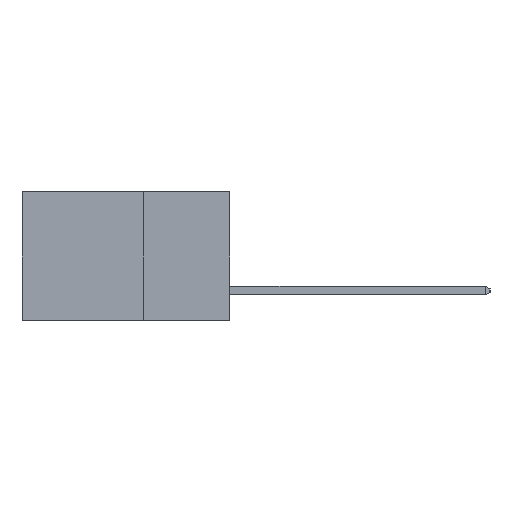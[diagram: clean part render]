
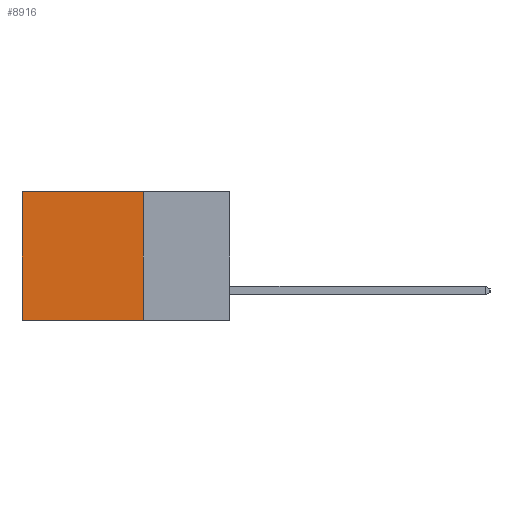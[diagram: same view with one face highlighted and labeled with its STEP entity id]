
A CAD part, left-side view. The second image highlights one B-rep face of the part: STEP entity #8916.
In plain terms, the highlighted planar face has unit normal (-1, 0, 0).
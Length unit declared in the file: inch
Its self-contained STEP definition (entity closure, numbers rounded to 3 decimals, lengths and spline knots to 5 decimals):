
#143 = DIRECTION ( 'NONE',  ( 0., 0., -1. ) ) ;
#251 = VERTEX_POINT ( 'NONE', #4258 ) ;
#1482 = EDGE_LOOP ( 'NONE', ( #3421, #2006, #2745, #1930 ) ) ;
#1563 = AXIS2_PLACEMENT_3D ( 'NONE', #13508, #4951, #7120 ) ;
#1855 = DIRECTION ( 'NONE',  ( 0., 1., 0. ) ) ;
#1930 = ORIENTED_EDGE ( 'NONE', *, *, #9659, .T. ) ;
#2006 = ORIENTED_EDGE ( 'NONE', *, *, #9370, .F. ) ;
#2319 = VECTOR ( 'NONE', #2576, 39.37008 ) ;
#2576 = DIRECTION ( 'NONE',  ( 0., 1., 0. ) ) ;
#2616 = VERTEX_POINT ( 'NONE', #10961 ) ;
#2745 = ORIENTED_EDGE ( 'NONE', *, *, #10788, .F. ) ;
#3421 = ORIENTED_EDGE ( 'NONE', *, *, #4397, .T. ) ;
#4176 = VECTOR ( 'NONE', #11426, 39.37008 ) ;
#4258 = CARTESIAN_POINT ( 'NONE',  ( 0.2615, 0.25, -0.37 ) ) ;
#4397 = EDGE_CURVE ( 'NONE', #7286, #8876, #6907, .T. ) ;
#4951 = DIRECTION ( 'NONE',  ( 1., 0., 0. ) ) ;
#4998 = LINE ( 'NONE', #6139, #13298 ) ;
#5422 = CARTESIAN_POINT ( 'NONE',  ( 0.2615, 0.6, -0.37 ) ) ;
#6139 = CARTESIAN_POINT ( 'NONE',  ( 0.2615, 0.25, 0. ) ) ;
#6532 = CARTESIAN_POINT ( 'NONE',  ( 0.2615, 0.25, -0.37 ) ) ;
#6907 = LINE ( 'NONE', #5422, #4176 ) ;
#7120 = DIRECTION ( 'NONE',  ( 0., 0., -1. ) ) ;
#7286 = VERTEX_POINT ( 'NONE', #9387 ) ;
#7936 = FACE_OUTER_BOUND ( 'NONE', #1482, .T. ) ;
#8876 = VERTEX_POINT ( 'NONE', #12491 ) ;
#8916 = ADVANCED_FACE ( 'NONE', ( #7936 ), #10298, .F. ) ;
#9370 = EDGE_CURVE ( 'NONE', #251, #8876, #10097, .T. ) ;
#9387 = CARTESIAN_POINT ( 'NONE',  ( 0.2615, 0.6, 0. ) ) ;
#9659 = EDGE_CURVE ( 'NONE', #2616, #7286, #4998, .T. ) ;
#10097 = LINE ( 'NONE', #11156, #2319 ) ;
#10298 = PLANE ( 'NONE',  #1563 ) ;
#10741 = VECTOR ( 'NONE', #143, 39.37008 ) ;
#10788 = EDGE_CURVE ( 'NONE', #2616, #251, #11918, .T. ) ;
#10961 = CARTESIAN_POINT ( 'NONE',  ( 0.2615, 0.25, 0. ) ) ;
#11156 = CARTESIAN_POINT ( 'NONE',  ( 0.2615, 0.25, -0.37 ) ) ;
#11426 = DIRECTION ( 'NONE',  ( 0., 0., -1. ) ) ;
#11918 = LINE ( 'NONE', #6532, #10741 ) ;
#12491 = CARTESIAN_POINT ( 'NONE',  ( 0.2615, 0.6, -0.37 ) ) ;
#13298 = VECTOR ( 'NONE', #1855, 39.37008 ) ;
#13508 = CARTESIAN_POINT ( 'NONE',  ( 0.2615, 0.25, -0.37 ) ) ;
